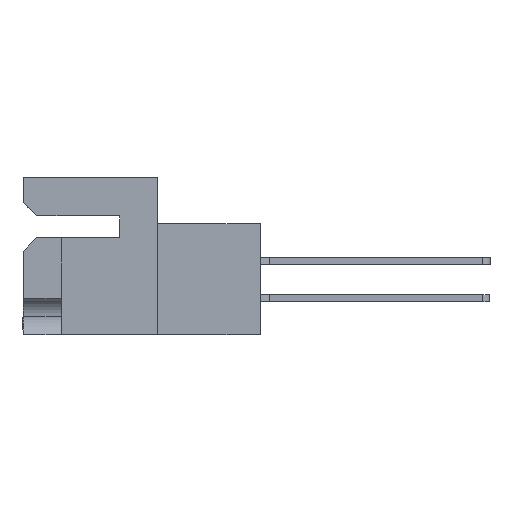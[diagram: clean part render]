
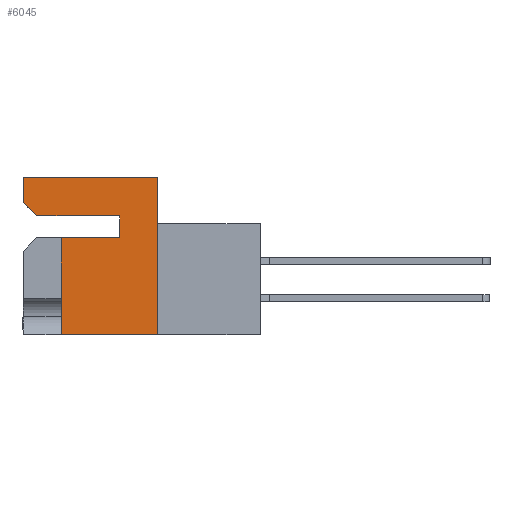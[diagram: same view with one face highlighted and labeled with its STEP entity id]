
A CAD part, left-side view. The second image highlights one B-rep face of the part: STEP entity #6045.
In plain terms, the highlighted planar face has unit normal (-1, 0, 0).
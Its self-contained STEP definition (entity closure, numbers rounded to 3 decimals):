
#797 = ORIENTED_EDGE ( 'NONE', *, *, #14028, .F. ) ;
#941 = CARTESIAN_POINT ( 'NONE',  ( 0., 8.255, -13.487 ) ) ;
#1081 = ORIENTED_EDGE ( 'NONE', *, *, #25794, .T. ) ;
#1378 = EDGE_CURVE ( 'NONE', #40063, #30854, #4760, .T. ) ;
#1601 = EDGE_CURVE ( 'NONE', #9538, #32145, #17524, .T. ) ;
#2115 = LINE ( 'NONE', #9131, #34562 ) ;
#2638 = VERTEX_POINT ( 'NONE', #16403 ) ;
#2642 = CARTESIAN_POINT ( 'NONE',  ( 0., -8.814, -13.487 ) ) ;
#2879 = EDGE_LOOP ( 'NONE', ( #15988, #12618, #797, #13855, #1081, #20927, #8513, #8372, #22886 ) ) ;
#3968 = CARTESIAN_POINT ( 'NONE',  ( 0., 0., -3.302 ) ) ;
#4183 = VERTEX_POINT ( 'NONE', #37867 ) ;
#4760 = LINE ( 'NONE', #33426, #13602 ) ;
#5659 = LINE ( 'NONE', #6004, #25863 ) ;
#5754 = DIRECTION ( 'NONE',  ( 0., -0.707, -0.707 ) ) ;
#6004 = CARTESIAN_POINT ( 'NONE',  ( 0., 10.363, -3.302 ) ) ;
#6045 = ADVANCED_FACE ( 'NONE', ( #39469 ), #10524, .F. ) ;
#6076 = LINE ( 'NONE', #13728, #31189 ) ;
#6566 = DIRECTION ( 'NONE',  ( 0., -1., 0. ) ) ;
#6600 = VECTOR ( 'NONE', #15479, 1000. ) ;
#8372 = ORIENTED_EDGE ( 'NONE', *, *, #1601, .F. ) ;
#8513 = ORIENTED_EDGE ( 'NONE', *, *, #23508, .F. ) ;
#9131 = CARTESIAN_POINT ( 'NONE',  ( 0., 3.251, -5.182 ) ) ;
#9198 = CARTESIAN_POINT ( 'NONE',  ( 0., 11.506, 0. ) ) ;
#9538 = VERTEX_POINT ( 'NONE', #27048 ) ;
#10442 = DIRECTION ( 'NONE',  ( 0., 0., 1. ) ) ;
#10473 = LINE ( 'NONE', #2642, #26656 ) ;
#10524 = PLANE ( 'NONE',  #27966 ) ;
#11738 = DIRECTION ( 'NONE',  ( 0., 0., 1. ) ) ;
#12618 = ORIENTED_EDGE ( 'NONE', *, *, #33747, .F. ) ;
#12677 = CARTESIAN_POINT ( 'NONE',  ( 0., 11.506, 0. ) ) ;
#13007 = LINE ( 'NONE', #9198, #6600 ) ;
#13602 = VECTOR ( 'NONE', #39587, 1000. ) ;
#13728 = CARTESIAN_POINT ( 'NONE',  ( 0., 8.255, -5.182 ) ) ;
#13855 = ORIENTED_EDGE ( 'NONE', *, *, #1378, .F. ) ;
#14028 = EDGE_CURVE ( 'NONE', #30854, #32384, #13007, .T. ) ;
#15432 = LINE ( 'NONE', #3968, #35143 ) ;
#15479 = DIRECTION ( 'NONE',  ( 0., -1., 0. ) ) ;
#15988 = ORIENTED_EDGE ( 'NONE', *, *, #37822, .F. ) ;
#16403 = CARTESIAN_POINT ( 'NONE',  ( 0., 3.251, -3.302 ) ) ;
#17361 = VERTEX_POINT ( 'NONE', #21043 ) ;
#17524 = LINE ( 'NONE', #22106, #25448 ) ;
#18071 = VERTEX_POINT ( 'NONE', #941 ) ;
#20453 = VECTOR ( 'NONE', #34503, 1000. ) ;
#20721 = CARTESIAN_POINT ( 'NONE',  ( 0., 11.506, -2.159 ) ) ;
#20927 = ORIENTED_EDGE ( 'NONE', *, *, #25953, .F. ) ;
#21043 = CARTESIAN_POINT ( 'NONE',  ( 0., 10.363, -3.302 ) ) ;
#21536 = CARTESIAN_POINT ( 'NONE',  ( 0., 0., 0. ) ) ;
#22106 = CARTESIAN_POINT ( 'NONE',  ( 0., 0., -5.182 ) ) ;
#22886 = ORIENTED_EDGE ( 'NONE', *, *, #35057, .F. ) ;
#23508 = EDGE_CURVE ( 'NONE', #32145, #2638, #2115, .T. ) ;
#25448 = VECTOR ( 'NONE', #6566, 1000. ) ;
#25794 = EDGE_CURVE ( 'NONE', #40063, #17361, #5659, .T. ) ;
#25863 = VECTOR ( 'NONE', #5754, 1000. ) ;
#25953 = EDGE_CURVE ( 'NONE', #2638, #17361, #15432, .T. ) ;
#26656 = VECTOR ( 'NONE', #37390, 1000. ) ;
#27048 = CARTESIAN_POINT ( 'NONE',  ( 0., 8.255, -5.182 ) ) ;
#27966 = AXIS2_PLACEMENT_3D ( 'NONE', #29738, #32790, #35664 ) ;
#28323 = CARTESIAN_POINT ( 'NONE',  ( 0., 0., 0. ) ) ;
#29738 = CARTESIAN_POINT ( 'NONE',  ( 0., 0., 0. ) ) ;
#30205 = CARTESIAN_POINT ( 'NONE',  ( 0., 3.251, -5.182 ) ) ;
#30854 = VERTEX_POINT ( 'NONE', #12677 ) ;
#31189 = VECTOR ( 'NONE', #10442, 1000. ) ;
#32145 = VERTEX_POINT ( 'NONE', #30205 ) ;
#32216 = LINE ( 'NONE', #28323, #20453 ) ;
#32384 = VERTEX_POINT ( 'NONE', #21536 ) ;
#32790 = DIRECTION ( 'NONE',  ( 1., 0., 0. ) ) ;
#33426 = CARTESIAN_POINT ( 'NONE',  ( 0., 11.506, -13.487 ) ) ;
#33747 = EDGE_CURVE ( 'NONE', #32384, #4183, #32216, .T. ) ;
#34503 = DIRECTION ( 'NONE',  ( 0., 0., -1. ) ) ;
#34562 = VECTOR ( 'NONE', #11738, 1000. ) ;
#35057 = EDGE_CURVE ( 'NONE', #18071, #9538, #6076, .T. ) ;
#35143 = VECTOR ( 'NONE', #38453, 1000. ) ;
#35664 = DIRECTION ( 'NONE',  ( 0., 0., -1. ) ) ;
#37390 = DIRECTION ( 'NONE',  ( 0., 1., 0. ) ) ;
#37822 = EDGE_CURVE ( 'NONE', #4183, #18071, #10473, .T. ) ;
#37867 = CARTESIAN_POINT ( 'NONE',  ( 0., 0., -13.487 ) ) ;
#38453 = DIRECTION ( 'NONE',  ( 0., 1., 0. ) ) ;
#39469 = FACE_OUTER_BOUND ( 'NONE', #2879, .T. ) ;
#39587 = DIRECTION ( 'NONE',  ( 0., 0., 1. ) ) ;
#40063 = VERTEX_POINT ( 'NONE', #20721 ) ;
